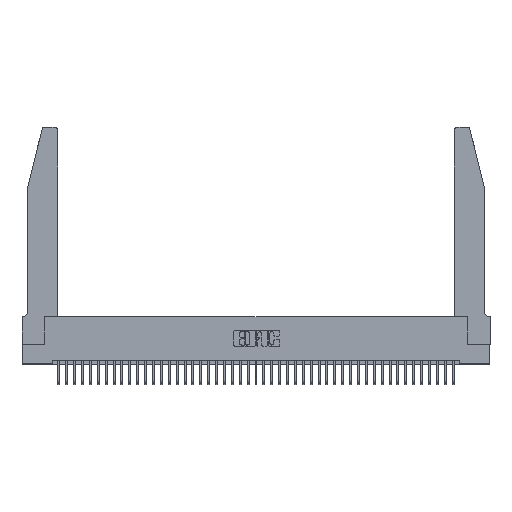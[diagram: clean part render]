
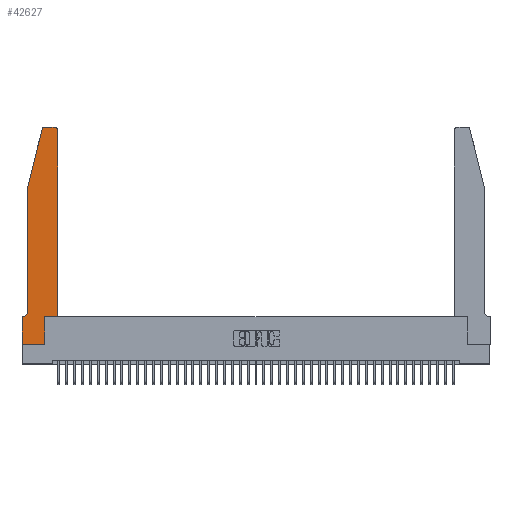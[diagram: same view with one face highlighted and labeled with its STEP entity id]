
A CAD part, top view. The second image highlights one B-rep face of the part: STEP entity #42627.
In plain terms, the highlighted planar face has unit normal (0, 0, 1).
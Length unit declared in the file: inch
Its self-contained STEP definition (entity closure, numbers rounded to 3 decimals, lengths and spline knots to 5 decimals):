
#219 = LINE ( 'NONE', #21769, #26196 ) ;
#506 = DIRECTION ( 'NONE',  ( 0., -1., 0. ) ) ;
#709 = EDGE_CURVE ( 'NONE', #44806, #42403, #23489, .T. ) ;
#713 = EDGE_CURVE ( 'NONE', #32536, #13721, #14161, .T. ) ;
#876 = ORIENTED_EDGE ( 'NONE', *, *, #30433, .T. ) ;
#1332 = DIRECTION ( 'NONE',  ( 1., 0., 0. ) ) ;
#2198 = ORIENTED_EDGE ( 'NONE', *, *, #37680, .T. ) ;
#2358 = CARTESIAN_POINT ( 'NONE',  ( 0.0055, 0.35, 0.37 ) ) ;
#3157 = CARTESIAN_POINT ( 'NONE',  ( 0., 0.35, 0.37 ) ) ;
#3926 = CARTESIAN_POINT ( 'NONE',  ( 0.284, 2.75, 0.37 ) ) ;
#3987 = VERTEX_POINT ( 'NONE', #28793 ) ;
#4172 = VERTEX_POINT ( 'NONE', #2358 ) ;
#4705 = VECTOR ( 'NONE', #7292, 39.37008 ) ;
#5408 = EDGE_CURVE ( 'NONE', #38466, #31575, #33672, .T. ) ;
#5523 = CARTESIAN_POINT ( 'NONE',  ( 0.0755, 0.35, 0.37 ) ) ;
#5762 = VECTOR ( 'NONE', #23287, 39.37008 ) ;
#6099 = EDGE_CURVE ( 'NONE', #15760, #17726, #36278, .T. ) ;
#6527 = EDGE_CURVE ( 'NONE', #17726, #38466, #17808, .T. ) ;
#6784 = PLANE ( 'NONE',  #17316 ) ;
#7292 = DIRECTION ( 'NONE',  ( 0., -1., 0. ) ) ;
#7514 = CIRCLE ( 'NONE', #32303, 0.03 ) ;
#9870 = CARTESIAN_POINT ( 'NONE',  ( 0.284, 2.72, 0.37 ) ) ;
#10336 = DIRECTION ( 'NONE',  ( 1., 0., 0. ) ) ;
#11473 = CARTESIAN_POINT ( 'NONE',  ( 0.4505, 0.35, 0.37 ) ) ;
#11989 = EDGE_CURVE ( 'NONE', #44699, #32536, #37814, .T. ) ;
#13441 = DIRECTION ( 'NONE',  ( 1., 0., 0. ) ) ;
#13721 = VERTEX_POINT ( 'NONE', #36459 ) ;
#13968 = CARTESIAN_POINT ( 'NONE',  ( 0.0055, 0.42, 0.37 ) ) ;
#14161 = LINE ( 'NONE', #17923, #31574 ) ;
#14219 = ORIENTED_EDGE ( 'NONE', *, *, #713, .T. ) ;
#14397 = DIRECTION ( 'NONE',  ( -0.239, -0.971, 0. ) ) ;
#15760 = VERTEX_POINT ( 'NONE', #40790 ) ;
#16049 = DIRECTION ( 'NONE',  ( -1., 0., 0. ) ) ;
#16284 = DIRECTION ( 'NONE',  ( 0., 1., 0. ) ) ;
#16390 = CARTESIAN_POINT ( 'NONE',  ( 0.4505, 0.35, 0.37 ) ) ;
#17114 = CARTESIAN_POINT ( 'NONE',  ( 0.4505, 0.35, 0.37 ) ) ;
#17221 = ORIENTED_EDGE ( 'NONE', *, *, #709, .T. ) ;
#17316 = AXIS2_PLACEMENT_3D ( 'NONE', #3157, #20675, #10336 ) ;
#17427 = CARTESIAN_POINT ( 'NONE',  ( 0.25487, 2.72718, 0.37 ) ) ;
#17503 = DIRECTION ( 'NONE',  ( -1., 0., 0. ) ) ;
#17726 = VERTEX_POINT ( 'NONE', #38207 ) ;
#17808 = LINE ( 'NONE', #11473, #35153 ) ;
#17923 = CARTESIAN_POINT ( 'NONE',  ( 0.0755, 2., 0.37 ) ) ;
#18448 = CARTESIAN_POINT ( 'NONE',  ( 0.4505, 2.72, 0.37 ) ) ;
#18571 = DIRECTION ( 'NONE',  ( 1., 0., 0. ) ) ;
#20675 = DIRECTION ( 'NONE',  ( 0., 0., 1. ) ) ;
#20932 = ORIENTED_EDGE ( 'NONE', *, *, #24499, .T. ) ;
#21769 = CARTESIAN_POINT ( 'NONE',  ( 0.0755, 2., 0.37 ) ) ;
#22337 = AXIS2_PLACEMENT_3D ( 'NONE', #9870, #34278, #13441 ) ;
#22568 = DIRECTION ( 'NONE',  ( 0., 0., 1. ) ) ;
#23287 = DIRECTION ( 'NONE',  ( 0., 1., 0. ) ) ;
#23479 = VECTOR ( 'NONE', #36967, 39.37008 ) ;
#23489 = LINE ( 'NONE', #31733, #4705 ) ;
#24499 = EDGE_CURVE ( 'NONE', #31575, #40970, #7514, .T. ) ;
#26196 = VECTOR ( 'NONE', #506, 39.37008 ) ;
#28793 = CARTESIAN_POINT ( 'NONE',  ( 0.0755, 0.42, 0.37 ) ) ;
#29309 = EDGE_CURVE ( 'NONE', #3987, #4172, #40270, .T. ) ;
#29712 = ORIENTED_EDGE ( 'NONE', *, *, #5408, .T. ) ;
#29836 = ORIENTED_EDGE ( 'NONE', *, *, #11989, .T. ) ;
#30127 = EDGE_CURVE ( 'NONE', #13721, #3987, #219, .T. ) ;
#30193 = CARTESIAN_POINT ( 'NONE',  ( 0., 0., 0.37 ) ) ;
#30433 = EDGE_CURVE ( 'NONE', #40970, #44699, #33754, .T. ) ;
#31021 = LINE ( 'NONE', #5523, #40161 ) ;
#31307 = ORIENTED_EDGE ( 'NONE', *, *, #6099, .T. ) ;
#31496 = VECTOR ( 'NONE', #33268, 39.37008 ) ;
#31574 = VECTOR ( 'NONE', #14397, 39.37008 ) ;
#31575 = VERTEX_POINT ( 'NONE', #18448 ) ;
#31733 = CARTESIAN_POINT ( 'NONE',  ( 0., 0., 0.37 ) ) ;
#32303 = AXIS2_PLACEMENT_3D ( 'NONE', #43180, #22568, #1332 ) ;
#32536 = VERTEX_POINT ( 'NONE', #17427 ) ;
#33117 = FACE_OUTER_BOUND ( 'NONE', #38381, .T. ) ;
#33268 = DIRECTION ( 'NONE',  ( 1., 0., 0. ) ) ;
#33672 = LINE ( 'NONE', #16390, #5762 ) ;
#33754 = LINE ( 'NONE', #40269, #23479 ) ;
#34278 = DIRECTION ( 'NONE',  ( 0., 0., 1. ) ) ;
#34517 = CARTESIAN_POINT ( 'NONE',  ( 0., 0.35, 0.37 ) ) ;
#35153 = VECTOR ( 'NONE', #18571, 39.37008 ) ;
#35196 = VECTOR ( 'NONE', #16284, 39.37008 ) ;
#35393 = CARTESIAN_POINT ( 'NONE',  ( 0.4205, 2.75, 0.37 ) ) ;
#36278 = LINE ( 'NONE', #40482, #35196 ) ;
#36369 = EDGE_CURVE ( 'NONE', #4172, #44806, #31021, .T. ) ;
#36459 = CARTESIAN_POINT ( 'NONE',  ( 0.0755, 2., 0.37 ) ) ;
#36551 = CARTESIAN_POINT ( 'NONE',  ( 0., 0., 0.37 ) ) ;
#36967 = DIRECTION ( 'NONE',  ( -1., 0., 0. ) ) ;
#37251 = ORIENTED_EDGE ( 'NONE', *, *, #36369, .T. ) ;
#37680 = EDGE_CURVE ( 'NONE', #42403, #15760, #41711, .T. ) ;
#37814 = CIRCLE ( 'NONE', #22337, 0.03 ) ;
#38198 = DIRECTION ( 'NONE',  ( 0., 0., -1. ) ) ;
#38207 = CARTESIAN_POINT ( 'NONE',  ( 0.2865, 0.35, 0.37 ) ) ;
#38381 = EDGE_LOOP ( 'NONE', ( #876, #29836, #14219, #41220, #39413, #37251, #17221, #2198, #31307, #43243, #29712, #20932 ) ) ;
#38466 = VERTEX_POINT ( 'NONE', #17114 ) ;
#39413 = ORIENTED_EDGE ( 'NONE', *, *, #29309, .T. ) ;
#40161 = VECTOR ( 'NONE', #16049, 39.37008 ) ;
#40269 = CARTESIAN_POINT ( 'NONE',  ( 0.2605, 2.75, 0.37 ) ) ;
#40270 = CIRCLE ( 'NONE', #43943, 0.07 ) ;
#40482 = CARTESIAN_POINT ( 'NONE',  ( 0.2865, 0.35, 0.37 ) ) ;
#40790 = CARTESIAN_POINT ( 'NONE',  ( 0.2865, 0., 0.37 ) ) ;
#40970 = VERTEX_POINT ( 'NONE', #35393 ) ;
#41220 = ORIENTED_EDGE ( 'NONE', *, *, #30127, .T. ) ;
#41711 = LINE ( 'NONE', #36551, #31496 ) ;
#42403 = VERTEX_POINT ( 'NONE', #30193 ) ;
#42627 = ADVANCED_FACE ( 'NONE', ( #33117 ), #6784, .T. ) ;
#43180 = CARTESIAN_POINT ( 'NONE',  ( 0.4205, 2.72, 0.37 ) ) ;
#43243 = ORIENTED_EDGE ( 'NONE', *, *, #6527, .T. ) ;
#43943 = AXIS2_PLACEMENT_3D ( 'NONE', #13968, #38198, #17503 ) ;
#44699 = VERTEX_POINT ( 'NONE', #3926 ) ;
#44806 = VERTEX_POINT ( 'NONE', #34517 ) ;
